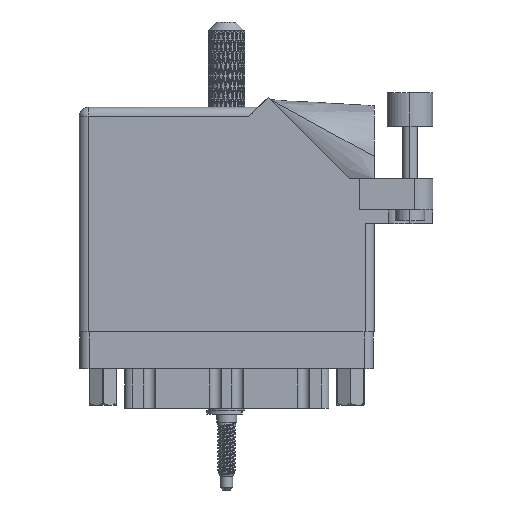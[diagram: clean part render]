
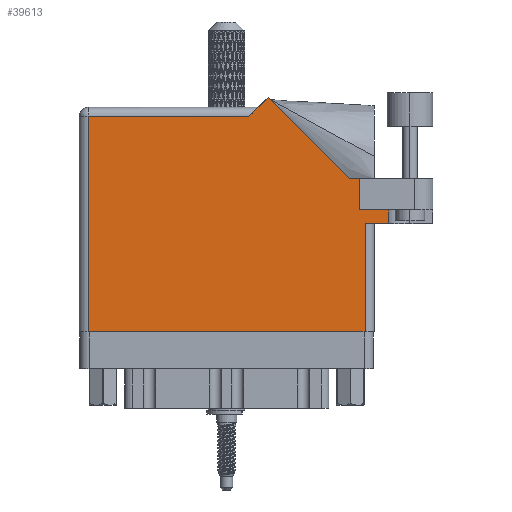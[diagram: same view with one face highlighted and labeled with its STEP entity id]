
A CAD part, front view. The second image highlights one B-rep face of the part: STEP entity #39613.
In plain terms, the highlighted face is planar.
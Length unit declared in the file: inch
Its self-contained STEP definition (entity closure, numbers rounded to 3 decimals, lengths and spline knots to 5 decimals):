
#285 = CARTESIAN_POINT ( 'NONE',  ( 0., 1.468, 0. ) ) ;
#2505 = ORIENTED_EDGE ( 'NONE', *, *, #66819, .T. ) ;
#2598 = FACE_OUTER_BOUND ( 'NONE', #21613, .T. ) ;
#3795 = VECTOR ( 'NONE', #93042, 39.37008 ) ;
#5530 = DIRECTION ( 'NONE',  ( 1., 0., 0. ) ) ;
#7201 = CARTESIAN_POINT ( 'NONE',  ( 1.91, 0.831, 0. ) ) ;
#9674 = DIRECTION ( 'NONE',  ( 0., 1., 0. ) ) ;
#11836 = VERTEX_POINT ( 'NONE', #34650 ) ;
#12184 = VERTEX_POINT ( 'NONE', #75347 ) ;
#12467 = DIRECTION ( 'NONE',  ( -0.707, 0.707, 0. ) ) ;
#13200 = VERTEX_POINT ( 'NONE', #99937 ) ;
#13450 = EDGE_CURVE ( 'NONE', #13200, #59149, #98656, .T. ) ;
#14900 = LINE ( 'NONE', #102214, #3795 ) ;
#16405 = LINE ( 'NONE', #42298, #42391 ) ;
#21362 = CARTESIAN_POINT ( 'NONE',  ( 1.948, 0.737, 0. ) ) ;
#21504 = VERTEX_POINT ( 'NONE', #100006 ) ;
#21613 = EDGE_LOOP ( 'NONE', ( #110857, #88660, #22108, #68737, #33637, #101919, #36662, #33293, #98918, #56237, #2505 ) ) ;
#22108 = ORIENTED_EDGE ( 'NONE', *, *, #49725, .T. ) ;
#23529 = EDGE_CURVE ( 'NONE', #83323, #35538, #80879, .T. ) ;
#29597 = CARTESIAN_POINT ( 'NONE',  ( 0.062, 1.468, 0. ) ) ;
#31428 = LINE ( 'NONE', #65854, #82553 ) ;
#33121 = VERTEX_POINT ( 'NONE', #29597 ) ;
#33293 = ORIENTED_EDGE ( 'NONE', *, *, #38218, .T. ) ;
#33637 = ORIENTED_EDGE ( 'NONE', *, *, #23529, .F. ) ;
#34517 = CARTESIAN_POINT ( 'NONE',  ( 2.1115, 1.16177, 0. ) ) ;
#34650 = CARTESIAN_POINT ( 'NONE',  ( 0.062, 0., 0. ) ) ;
#35114 = VECTOR ( 'NONE', #95376, 39.37008 ) ;
#35538 = VERTEX_POINT ( 'NONE', #107343 ) ;
#35923 = CARTESIAN_POINT ( 'NONE',  ( 1.84442, 1.044, 0. ) ) ;
#36662 = ORIENTED_EDGE ( 'NONE', *, *, #72190, .T. ) ;
#37224 = VECTOR ( 'NONE', #9674, 39.37008 ) ;
#38218 = EDGE_CURVE ( 'NONE', #48771, #12184, #31428, .T. ) ;
#39613 = ADVANCED_FACE ( 'NONE', ( #2598 ), #62912, .F. ) ;
#42298 = CARTESIAN_POINT ( 'NONE',  ( 2.01, 0.737, 0. ) ) ;
#42391 = VECTOR ( 'NONE', #5530, 39.37008 ) ;
#42848 = LINE ( 'NONE', #68677, #90786 ) ;
#44175 = CARTESIAN_POINT ( 'NONE',  ( 1.948, 0.737, 0. ) ) ;
#45820 = CARTESIAN_POINT ( 'NONE',  ( 2.1115, 0.737, 0. ) ) ;
#46645 = CARTESIAN_POINT ( 'NONE',  ( 1.155, 1.468, 0. ) ) ;
#48771 = VERTEX_POINT ( 'NONE', #35923 ) ;
#49243 = VECTOR ( 'NONE', #74429, 39.37008 ) ;
#49725 = EDGE_CURVE ( 'NONE', #59149, #106295, #16405, .T. ) ;
#52459 = EDGE_CURVE ( 'NONE', #82310, #33121, #95630, .T. ) ;
#53220 = EDGE_CURVE ( 'NONE', #83323, #21504, #42848, .T. ) ;
#55346 = DIRECTION ( 'NONE',  ( -1., 0., 0. ) ) ;
#55450 = DIRECTION ( 'NONE',  ( -1., 0., 0. ) ) ;
#56237 = ORIENTED_EDGE ( 'NONE', *, *, #52459, .T. ) ;
#59149 = VERTEX_POINT ( 'NONE', #21362 ) ;
#62613 = EDGE_CURVE ( 'NONE', #35538, #106295, #67833, .T. ) ;
#62912 = PLANE ( 'NONE',  #80912 ) ;
#63225 = VECTOR ( 'NONE', #70357, 39.37008 ) ;
#65854 = CARTESIAN_POINT ( 'NONE',  ( 1.84442, 1.044, 0. ) ) ;
#66819 = EDGE_CURVE ( 'NONE', #33121, #11836, #14900, .T. ) ;
#67833 = LINE ( 'NONE', #34517, #35114 ) ;
#68677 = CARTESIAN_POINT ( 'NONE',  ( 1.91, 0.831, 0. ) ) ;
#68737 = ORIENTED_EDGE ( 'NONE', *, *, #62613, .F. ) ;
#70357 = DIRECTION ( 'NONE',  ( -1., 0., 0. ) ) ;
#72190 = EDGE_CURVE ( 'NONE', #21504, #48771, #89777, .T. ) ;
#74429 = DIRECTION ( 'NONE',  ( 1., 0., 0. ) ) ;
#75347 = CARTESIAN_POINT ( 'NONE',  ( 1.28771, 1.60071, 0. ) ) ;
#75830 = EDGE_CURVE ( 'NONE', #11836, #13200, #108285, .T. ) ;
#77242 = LINE ( 'NONE', #103634, #79599 ) ;
#79599 = VECTOR ( 'NONE', #95041, 39.37008 ) ;
#80316 = CARTESIAN_POINT ( 'NONE',  ( 1.91, 0.831, 0. ) ) ;
#80879 = LINE ( 'NONE', #80316, #92202 ) ;
#80912 = AXIS2_PLACEMENT_3D ( 'NONE', #89885, #97951, #55450 ) ;
#82310 = VERTEX_POINT ( 'NONE', #46645 ) ;
#82553 = VECTOR ( 'NONE', #12467, 39.37008 ) ;
#83323 = VERTEX_POINT ( 'NONE', #7201 ) ;
#88660 = ORIENTED_EDGE ( 'NONE', *, *, #13450, .T. ) ;
#89229 = CARTESIAN_POINT ( 'NONE',  ( 2.41, 1.044, 0. ) ) ;
#89777 = LINE ( 'NONE', #89229, #103234 ) ;
#89885 = CARTESIAN_POINT ( 'NONE',  ( 0., 1.53, 0. ) ) ;
#90786 = VECTOR ( 'NONE', #103692, 39.37008 ) ;
#91630 = CARTESIAN_POINT ( 'NONE',  ( 0., 0., 0. ) ) ;
#92202 = VECTOR ( 'NONE', #106144, 39.37008 ) ;
#93042 = DIRECTION ( 'NONE',  ( 0., -1., 0. ) ) ;
#95041 = DIRECTION ( 'NONE',  ( -0.707, -0.707, 0. ) ) ;
#95376 = DIRECTION ( 'NONE',  ( 0., -1., 0. ) ) ;
#95630 = LINE ( 'NONE', #285, #63225 ) ;
#96364 = EDGE_CURVE ( 'NONE', #12184, #82310, #77242, .T. ) ;
#97951 = DIRECTION ( 'NONE',  ( 0., 0., -1. ) ) ;
#98656 = LINE ( 'NONE', #44175, #37224 ) ;
#98918 = ORIENTED_EDGE ( 'NONE', *, *, #96364, .T. ) ;
#99937 = CARTESIAN_POINT ( 'NONE',  ( 1.948, 0., 0. ) ) ;
#100006 = CARTESIAN_POINT ( 'NONE',  ( 1.91, 1.044, 0. ) ) ;
#101919 = ORIENTED_EDGE ( 'NONE', *, *, #53220, .T. ) ;
#102214 = CARTESIAN_POINT ( 'NONE',  ( 0.062, 0., 0. ) ) ;
#103234 = VECTOR ( 'NONE', #55346, 39.37008 ) ;
#103634 = CARTESIAN_POINT ( 'NONE',  ( 1.217, 1.53, 0. ) ) ;
#103692 = DIRECTION ( 'NONE',  ( 0., 1., 0. ) ) ;
#106144 = DIRECTION ( 'NONE',  ( 1., 0., 0. ) ) ;
#106295 = VERTEX_POINT ( 'NONE', #45820 ) ;
#107343 = CARTESIAN_POINT ( 'NONE',  ( 2.1115, 0.831, 0. ) ) ;
#108285 = LINE ( 'NONE', #91630, #49243 ) ;
#110857 = ORIENTED_EDGE ( 'NONE', *, *, #75830, .T. ) ;
